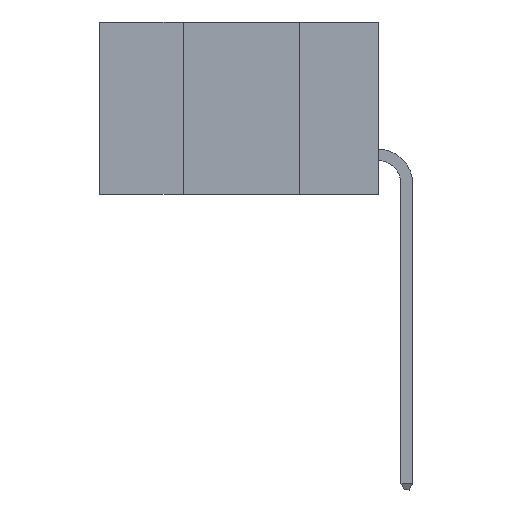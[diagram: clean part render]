
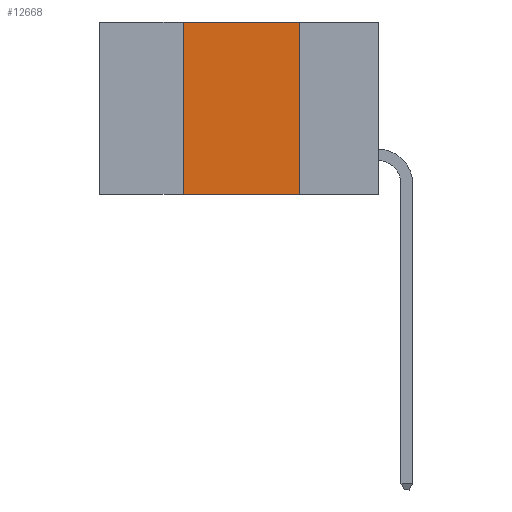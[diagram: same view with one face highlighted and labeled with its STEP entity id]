
A CAD part, left-side view. The second image highlights one B-rep face of the part: STEP entity #12668.
In plain terms, the highlighted planar face has unit normal (-1, 0, 0).
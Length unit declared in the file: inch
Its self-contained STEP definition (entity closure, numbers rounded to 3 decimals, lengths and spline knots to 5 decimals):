
#459 = VECTOR ( 'NONE', #1960, 39.37008 ) ;
#1175 = DIRECTION ( 'NONE',  ( 1., 0., 0. ) ) ;
#1394 = EDGE_CURVE ( 'NONE', #3564, #3759, #11619, .T. ) ;
#1602 = LINE ( 'NONE', #14079, #7544 ) ;
#1725 = VERTEX_POINT ( 'NONE', #10116 ) ;
#1960 = DIRECTION ( 'NONE',  ( 0., 0., 1. ) ) ;
#2648 = EDGE_LOOP ( 'NONE', ( #11064, #14700, #13640, #14411 ) ) ;
#2793 = LINE ( 'NONE', #7691, #14640 ) ;
#3026 = DIRECTION ( 'NONE',  ( 0., -1., 0. ) ) ;
#3564 = VERTEX_POINT ( 'NONE', #4226 ) ;
#3675 = LINE ( 'NONE', #7829, #459 ) ;
#3759 = VERTEX_POINT ( 'NONE', #10399 ) ;
#4226 = CARTESIAN_POINT ( 'NONE',  ( 0., 0.17, 0. ) ) ;
#5802 = DIRECTION ( 'NONE',  ( 0., -1., 0. ) ) ;
#6819 = CARTESIAN_POINT ( 'NONE',  ( 0., 0.17, 0. ) ) ;
#7148 = PLANE ( 'NONE',  #8295 ) ;
#7446 = DIRECTION ( 'NONE',  ( 0., 0., -1. ) ) ;
#7544 = VECTOR ( 'NONE', #5802, 39.37008 ) ;
#7691 = CARTESIAN_POINT ( 'NONE',  ( 0., 0.6, 0. ) ) ;
#7829 = CARTESIAN_POINT ( 'NONE',  ( 0., 0.42, 0. ) ) ;
#8295 = AXIS2_PLACEMENT_3D ( 'NONE', #15437, #1175, #9412 ) ;
#9412 = DIRECTION ( 'NONE',  ( 0., 0., -1. ) ) ;
#10116 = CARTESIAN_POINT ( 'NONE',  ( 0., 0.42, 0. ) ) ;
#10270 = EDGE_CURVE ( 'NONE', #1725, #3564, #2793, .T. ) ;
#10399 = CARTESIAN_POINT ( 'NONE',  ( 0., 0.17, -0.37 ) ) ;
#11064 = ORIENTED_EDGE ( 'NONE', *, *, #1394, .F. ) ;
#11205 = EDGE_CURVE ( 'NONE', #15049, #3759, #1602, .T. ) ;
#11251 = VECTOR ( 'NONE', #7446, 39.37008 ) ;
#11619 = LINE ( 'NONE', #6819, #11251 ) ;
#12668 = ADVANCED_FACE ( 'NONE', ( #13688 ), #7148, .F. ) ;
#12948 = CARTESIAN_POINT ( 'NONE',  ( 0., 0.42, -0.37 ) ) ;
#13636 = EDGE_CURVE ( 'NONE', #15049, #1725, #3675, .T. ) ;
#13640 = ORIENTED_EDGE ( 'NONE', *, *, #13636, .F. ) ;
#13688 = FACE_OUTER_BOUND ( 'NONE', #2648, .T. ) ;
#14079 = CARTESIAN_POINT ( 'NONE',  ( 0., 0.6, -0.37 ) ) ;
#14411 = ORIENTED_EDGE ( 'NONE', *, *, #11205, .T. ) ;
#14640 = VECTOR ( 'NONE', #3026, 39.37008 ) ;
#14700 = ORIENTED_EDGE ( 'NONE', *, *, #10270, .F. ) ;
#15049 = VERTEX_POINT ( 'NONE', #12948 ) ;
#15437 = CARTESIAN_POINT ( 'NONE',  ( 0., 0.6, 0. ) ) ;
